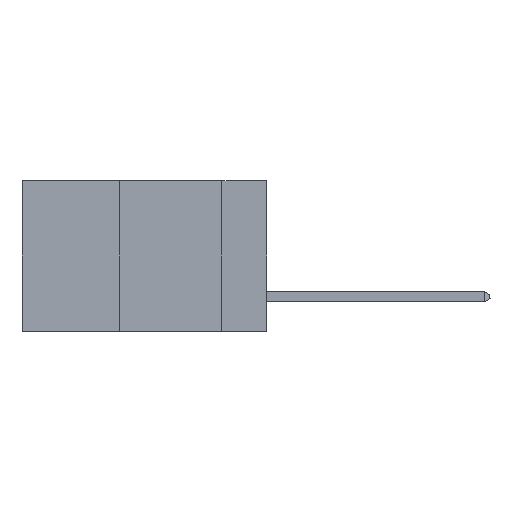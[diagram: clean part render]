
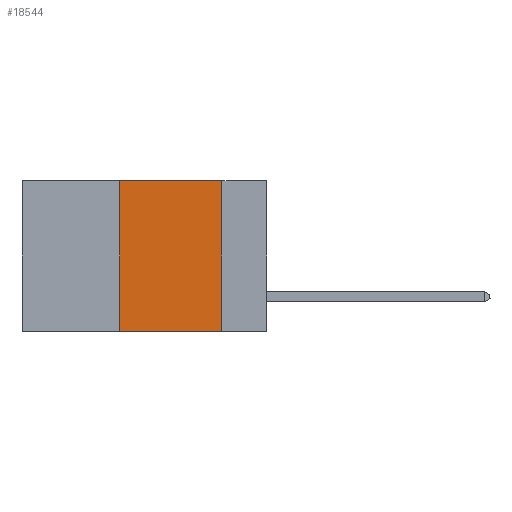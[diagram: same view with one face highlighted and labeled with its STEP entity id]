
A CAD part, left-side view. The second image highlights one B-rep face of the part: STEP entity #18544.
In plain terms, the highlighted planar face has unit normal (-1, 0, 0).
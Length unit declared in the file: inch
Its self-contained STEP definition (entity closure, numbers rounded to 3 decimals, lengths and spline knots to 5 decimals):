
#337 = ORIENTED_EDGE ( 'NONE', *, *, #2065, .F. ) ;
#1595 = LINE ( 'NONE', #18242, #13953 ) ;
#2065 = EDGE_CURVE ( 'NONE', #11941, #21157, #19762, .T. ) ;
#2535 = DIRECTION ( 'NONE',  ( 0., -1., 0. ) ) ;
#4190 = CARTESIAN_POINT ( 'NONE',  ( 0., 0.36, 0. ) ) ;
#4561 = ORIENTED_EDGE ( 'NONE', *, *, #14731, .T. ) ;
#4779 = DIRECTION ( 'NONE',  ( 1., 0., 0. ) ) ;
#5065 = VECTOR ( 'NONE', #13442, 39.37008 ) ;
#6244 = ORIENTED_EDGE ( 'NONE', *, *, #11286, .F. ) ;
#6459 = VECTOR ( 'NONE', #22076, 39.37008 ) ;
#6706 = AXIS2_PLACEMENT_3D ( 'NONE', #10104, #4779, #15939 ) ;
#8762 = CARTESIAN_POINT ( 'NONE',  ( 0., 0.11, 0. ) ) ;
#10030 = PLANE ( 'NONE',  #6706 ) ;
#10104 = CARTESIAN_POINT ( 'NONE',  ( 0., 0.6, 0. ) ) ;
#10435 = CARTESIAN_POINT ( 'NONE',  ( 0., 0.36, -0.37 ) ) ;
#11284 = ORIENTED_EDGE ( 'NONE', *, *, #15456, .F. ) ;
#11286 = EDGE_CURVE ( 'NONE', #14357, #17489, #18237, .T. ) ;
#11321 = VECTOR ( 'NONE', #2535, 39.37008 ) ;
#11941 = VERTEX_POINT ( 'NONE', #10435 ) ;
#13442 = DIRECTION ( 'NONE',  ( 0., 0., 1. ) ) ;
#13953 = VECTOR ( 'NONE', #16521, 39.37008 ) ;
#14357 = VERTEX_POINT ( 'NONE', #15972 ) ;
#14731 = EDGE_CURVE ( 'NONE', #11941, #17489, #16035, .T. ) ;
#15456 = EDGE_CURVE ( 'NONE', #21157, #14357, #1595, .T. ) ;
#15939 = DIRECTION ( 'NONE',  ( 0., 0., -1. ) ) ;
#15972 = CARTESIAN_POINT ( 'NONE',  ( 0., 0.11, 0. ) ) ;
#16035 = LINE ( 'NONE', #23395, #11321 ) ;
#16521 = DIRECTION ( 'NONE',  ( 0., -1., 0. ) ) ;
#17489 = VERTEX_POINT ( 'NONE', #19024 ) ;
#18237 = LINE ( 'NONE', #8762, #6459 ) ;
#18242 = CARTESIAN_POINT ( 'NONE',  ( 0., 0.6, 0. ) ) ;
#18544 = ADVANCED_FACE ( 'NONE', ( #19279 ), #10030, .F. ) ;
#19024 = CARTESIAN_POINT ( 'NONE',  ( 0., 0.11, -0.37 ) ) ;
#19279 = FACE_OUTER_BOUND ( 'NONE', #23531, .T. ) ;
#19762 = LINE ( 'NONE', #4190, #5065 ) ;
#21157 = VERTEX_POINT ( 'NONE', #22359 ) ;
#22076 = DIRECTION ( 'NONE',  ( 0., 0., -1. ) ) ;
#22359 = CARTESIAN_POINT ( 'NONE',  ( 0., 0.36, 0. ) ) ;
#23395 = CARTESIAN_POINT ( 'NONE',  ( 0., 0.6, -0.37 ) ) ;
#23531 = EDGE_LOOP ( 'NONE', ( #6244, #11284, #337, #4561 ) ) ;
